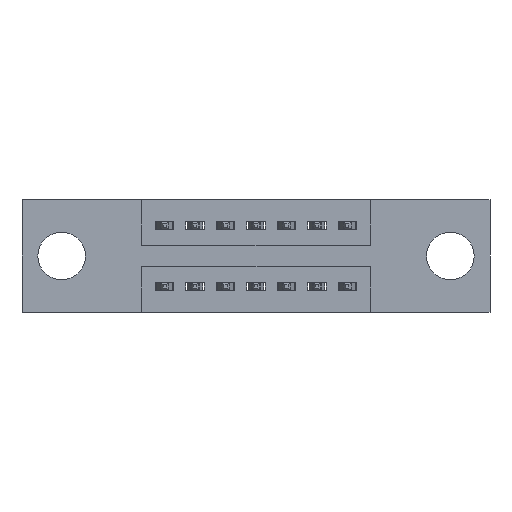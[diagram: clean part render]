
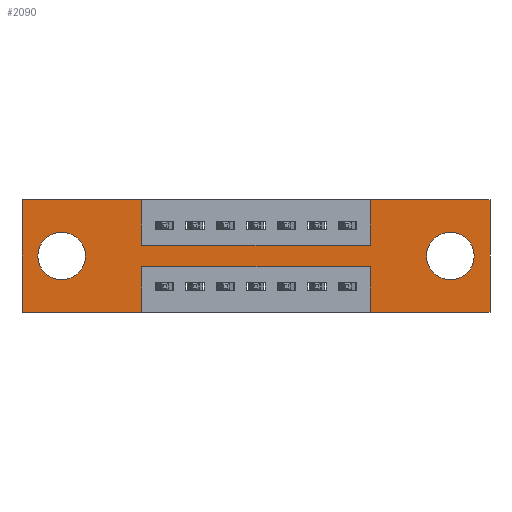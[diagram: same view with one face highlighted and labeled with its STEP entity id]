
A CAD part, front view. The second image highlights one B-rep face of the part: STEP entity #2090.
In plain terms, the highlighted planar face has unit normal (0, -1, 0).
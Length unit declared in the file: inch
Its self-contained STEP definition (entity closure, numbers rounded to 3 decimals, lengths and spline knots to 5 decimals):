
#34 = CARTESIAN_POINT ( 'NONE',  ( 1.535, 0., -0.37 ) ) ;
#132 = EDGE_CURVE ( 'NONE', #414, #5168, #3600, .T. ) ;
#209 = EDGE_CURVE ( 'NONE', #4114, #6818, #6439, .T. ) ;
#267 = DIRECTION ( 'NONE',  ( -1., 0., 0. ) ) ;
#304 = VECTOR ( 'NONE', #3196, 39.37008 ) ;
#315 = DIRECTION ( 'NONE',  ( 0., 0., 1. ) ) ;
#351 = EDGE_CURVE ( 'NONE', #9634, #5052, #2243, .T. ) ;
#364 = AXIS2_PLACEMENT_3D ( 'NONE', #789, #4036, #864 ) ;
#379 = FACE_OUTER_BOUND ( 'NONE', #1907, .T. ) ;
#414 = VERTEX_POINT ( 'NONE', #6142 ) ;
#538 = CARTESIAN_POINT ( 'NONE',  ( 1.1425, 0., 0. ) ) ;
#718 = DIRECTION ( 'NONE',  ( 0., -1., 0. ) ) ;
#789 = CARTESIAN_POINT ( 'NONE',  ( 1.405, 0., -0.185 ) ) ;
#864 = DIRECTION ( 'NONE',  ( 0., 0., -1. ) ) ;
#882 = LINE ( 'NONE', #5283, #1982 ) ;
#901 = DIRECTION ( 'NONE',  ( 0., 1., 0. ) ) ;
#1077 = DIRECTION ( 'NONE',  ( 0., 1., 0. ) ) ;
#1159 = CARTESIAN_POINT ( 'NONE',  ( 0., 0., 0. ) ) ;
#1288 = VECTOR ( 'NONE', #267, 39.37008 ) ;
#1500 = FACE_BOUND ( 'NONE', #8549, .T. ) ;
#1506 = ORIENTED_EDGE ( 'NONE', *, *, #9009, .F. ) ;
#1632 = DIRECTION ( 'NONE',  ( 0., 0., -1. ) ) ;
#1660 = DIRECTION ( 'NONE',  ( 1., 0., 0. ) ) ;
#1853 = CARTESIAN_POINT ( 'NONE',  ( 0.13, 0., -0.185 ) ) ;
#1865 = VECTOR ( 'NONE', #4232, 39.37008 ) ;
#1907 = EDGE_LOOP ( 'NONE', ( #6848, #4354, #9136, #1506, #6352, #5959, #7823, #7233, #10122, #5126, #6548, #6002 ) ) ;
#1982 = VECTOR ( 'NONE', #8779, 39.37008 ) ;
#2044 = LINE ( 'NONE', #6626, #3016 ) ;
#2090 = ADVANCED_FACE ( 'NONE', ( #1500, #10137, #379 ), #10070, .T. ) ;
#2243 = LINE ( 'NONE', #4382, #8785 ) ;
#2335 = CARTESIAN_POINT ( 'NONE',  ( 0.3925, 0., 0. ) ) ;
#2374 = CARTESIAN_POINT ( 'NONE',  ( 1.1425, 0., -0.37 ) ) ;
#2395 = CARTESIAN_POINT ( 'NONE',  ( 1.1425, 0., -0.22 ) ) ;
#2515 = ORIENTED_EDGE ( 'NONE', *, *, #132, .T. ) ;
#2697 = DIRECTION ( 'NONE',  ( 0., 0., 1. ) ) ;
#2710 = CARTESIAN_POINT ( 'NONE',  ( 0.3925, 0., -0.15 ) ) ;
#2835 = CARTESIAN_POINT ( 'NONE',  ( 1.405, 0., -0.263 ) ) ;
#2927 = CIRCLE ( 'NONE', #6636, 0.078 ) ;
#3016 = VECTOR ( 'NONE', #5797, 39.37008 ) ;
#3147 = DIRECTION ( 'NONE',  ( 0., 0., -1. ) ) ;
#3196 = DIRECTION ( 'NONE',  ( 0., 0., 1. ) ) ;
#3208 = LINE ( 'NONE', #3765, #9414 ) ;
#3282 = CIRCLE ( 'NONE', #4840, 0.078 ) ;
#3320 = EDGE_CURVE ( 'NONE', #4879, #5774, #9373, .T. ) ;
#3321 = ORIENTED_EDGE ( 'NONE', *, *, #3840, .T. ) ;
#3591 = LINE ( 'NONE', #8186, #1865 ) ;
#3600 = CIRCLE ( 'NONE', #364, 0.078 ) ;
#3765 = CARTESIAN_POINT ( 'NONE',  ( 0.3925, 0., -0.37 ) ) ;
#3837 = CARTESIAN_POINT ( 'NONE',  ( 0., 0., -0.37 ) ) ;
#3840 = EDGE_CURVE ( 'NONE', #7845, #9971, #7763, .T. ) ;
#3942 = VECTOR ( 'NONE', #9402, 39.37008 ) ;
#3985 = EDGE_CURVE ( 'NONE', #5052, #7646, #9267, .T. ) ;
#4036 = DIRECTION ( 'NONE',  ( 0., 1., 0. ) ) ;
#4043 = ORIENTED_EDGE ( 'NONE', *, *, #4111, .T. ) ;
#4089 = ORIENTED_EDGE ( 'NONE', *, *, #4221, .T. ) ;
#4111 = EDGE_CURVE ( 'NONE', #5168, #414, #3282, .T. ) ;
#4114 = VERTEX_POINT ( 'NONE', #2395 ) ;
#4116 = CARTESIAN_POINT ( 'NONE',  ( 0.3925, 0., -0.22 ) ) ;
#4207 = EDGE_CURVE ( 'NONE', #5157, #8251, #6505, .T. ) ;
#4221 = EDGE_CURVE ( 'NONE', #9971, #7845, #2927, .T. ) ;
#4232 = DIRECTION ( 'NONE',  ( -1., 0., 0. ) ) ;
#4273 = VECTOR ( 'NONE', #1660, 39.37008 ) ;
#4354 = ORIENTED_EDGE ( 'NONE', *, *, #209, .F. ) ;
#4382 = CARTESIAN_POINT ( 'NONE',  ( 0., 0., -0.37 ) ) ;
#4459 = EDGE_CURVE ( 'NONE', #8251, #7363, #5123, .T. ) ;
#4523 = VECTOR ( 'NONE', #2697, 39.37008 ) ;
#4783 = DIRECTION ( 'NONE',  ( 0., 1., 0. ) ) ;
#4819 = CARTESIAN_POINT ( 'NONE',  ( 0.3925, 0., -0.15 ) ) ;
#4840 = AXIS2_PLACEMENT_3D ( 'NONE', #5574, #901, #6359 ) ;
#4864 = CARTESIAN_POINT ( 'NONE',  ( 0.13, 0., -0.107 ) ) ;
#4879 = VERTEX_POINT ( 'NONE', #5333 ) ;
#4888 = VERTEX_POINT ( 'NONE', #538 ) ;
#5052 = VERTEX_POINT ( 'NONE', #5857 ) ;
#5090 = EDGE_CURVE ( 'NONE', #7363, #4888, #2044, .T. ) ;
#5123 = LINE ( 'NONE', #4819, #4273 ) ;
#5126 = ORIENTED_EDGE ( 'NONE', *, *, #8133, .F. ) ;
#5139 = CARTESIAN_POINT ( 'NONE',  ( 0.3925, 0., -0.22 ) ) ;
#5157 = VERTEX_POINT ( 'NONE', #9013 ) ;
#5168 = VERTEX_POINT ( 'NONE', #2835 ) ;
#5258 = DIRECTION ( 'NONE',  ( 0., 0., -1. ) ) ;
#5283 = CARTESIAN_POINT ( 'NONE',  ( 0., 0., 0. ) ) ;
#5333 = CARTESIAN_POINT ( 'NONE',  ( 1.535, 0., 0. ) ) ;
#5454 = CARTESIAN_POINT ( 'NONE',  ( 0., 0., 0. ) ) ;
#5479 = DIRECTION ( 'NONE',  ( 0., 0., -1. ) ) ;
#5574 = CARTESIAN_POINT ( 'NONE',  ( 1.405, 0., -0.185 ) ) ;
#5693 = DIRECTION ( 'NONE',  ( 0., 0., 1. ) ) ;
#5774 = VERTEX_POINT ( 'NONE', #34 ) ;
#5797 = DIRECTION ( 'NONE',  ( 0., 0., 1. ) ) ;
#5812 = EDGE_CURVE ( 'NONE', #7054, #4114, #6093, .T. ) ;
#5857 = CARTESIAN_POINT ( 'NONE',  ( 0., 0., -0.37 ) ) ;
#5890 = CARTESIAN_POINT ( 'NONE',  ( 0.3925, 0., -0.37 ) ) ;
#5959 = ORIENTED_EDGE ( 'NONE', *, *, #9183, .F. ) ;
#6002 = ORIENTED_EDGE ( 'NONE', *, *, #351, .F. ) ;
#6093 = LINE ( 'NONE', #2374, #304 ) ;
#6142 = CARTESIAN_POINT ( 'NONE',  ( 1.405, 0., -0.107 ) ) ;
#6178 = AXIS2_PLACEMENT_3D ( 'NONE', #8085, #4783, #315 ) ;
#6302 = LINE ( 'NONE', #7826, #3942 ) ;
#6352 = ORIENTED_EDGE ( 'NONE', *, *, #3320, .F. ) ;
#6359 = DIRECTION ( 'NONE',  ( 0., 0., -1. ) ) ;
#6439 = LINE ( 'NONE', #4116, #1288 ) ;
#6505 = LINE ( 'NONE', #2335, #9138 ) ;
#6548 = ORIENTED_EDGE ( 'NONE', *, *, #3985, .F. ) ;
#6626 = CARTESIAN_POINT ( 'NONE',  ( 1.1425, 0., 0. ) ) ;
#6636 = AXIS2_PLACEMENT_3D ( 'NONE', #1853, #1077, #5693 ) ;
#6818 = VERTEX_POINT ( 'NONE', #5139 ) ;
#6848 = ORIENTED_EDGE ( 'NONE', *, *, #9260, .F. ) ;
#7054 = VERTEX_POINT ( 'NONE', #9394 ) ;
#7233 = ORIENTED_EDGE ( 'NONE', *, *, #4459, .F. ) ;
#7363 = VERTEX_POINT ( 'NONE', #8159 ) ;
#7420 = DIRECTION ( 'NONE',  ( -1., 0., 0. ) ) ;
#7646 = VERTEX_POINT ( 'NONE', #5454 ) ;
#7743 = VECTOR ( 'NONE', #5258, 39.37008 ) ;
#7763 = CIRCLE ( 'NONE', #6178, 0.078 ) ;
#7823 = ORIENTED_EDGE ( 'NONE', *, *, #5090, .F. ) ;
#7826 = CARTESIAN_POINT ( 'NONE',  ( 0., 0., 0. ) ) ;
#7845 = VERTEX_POINT ( 'NONE', #4864 ) ;
#7900 = AXIS2_PLACEMENT_3D ( 'NONE', #3837, #718, #3147 ) ;
#8085 = CARTESIAN_POINT ( 'NONE',  ( 0.13, 0., -0.185 ) ) ;
#8133 = EDGE_CURVE ( 'NONE', #7646, #5157, #882, .T. ) ;
#8159 = CARTESIAN_POINT ( 'NONE',  ( 1.1425, 0., -0.15 ) ) ;
#8186 = CARTESIAN_POINT ( 'NONE',  ( 0., 0., -0.37 ) ) ;
#8251 = VERTEX_POINT ( 'NONE', #2710 ) ;
#8470 = CARTESIAN_POINT ( 'NONE',  ( 0.13, 0., -0.263 ) ) ;
#8496 = EDGE_LOOP ( 'NONE', ( #3321, #4089 ) ) ;
#8549 = EDGE_LOOP ( 'NONE', ( #2515, #4043 ) ) ;
#8779 = DIRECTION ( 'NONE',  ( 1., 0., 0. ) ) ;
#8785 = VECTOR ( 'NONE', #7420, 39.37008 ) ;
#9009 = EDGE_CURVE ( 'NONE', #5774, #7054, #3591, .T. ) ;
#9013 = CARTESIAN_POINT ( 'NONE',  ( 0.3925, 0., 0. ) ) ;
#9136 = ORIENTED_EDGE ( 'NONE', *, *, #5812, .F. ) ;
#9138 = VECTOR ( 'NONE', #1632, 39.37008 ) ;
#9183 = EDGE_CURVE ( 'NONE', #4888, #4879, #6302, .T. ) ;
#9220 = CARTESIAN_POINT ( 'NONE',  ( 1.535, 0., 0. ) ) ;
#9260 = EDGE_CURVE ( 'NONE', #6818, #9634, #3208, .T. ) ;
#9267 = LINE ( 'NONE', #1159, #4523 ) ;
#9373 = LINE ( 'NONE', #9220, #7743 ) ;
#9394 = CARTESIAN_POINT ( 'NONE',  ( 1.1425, 0., -0.37 ) ) ;
#9402 = DIRECTION ( 'NONE',  ( 1., 0., 0. ) ) ;
#9414 = VECTOR ( 'NONE', #5479, 39.37008 ) ;
#9634 = VERTEX_POINT ( 'NONE', #5890 ) ;
#9971 = VERTEX_POINT ( 'NONE', #8470 ) ;
#10070 = PLANE ( 'NONE',  #7900 ) ;
#10122 = ORIENTED_EDGE ( 'NONE', *, *, #4207, .F. ) ;
#10137 = FACE_BOUND ( 'NONE', #8496, .T. ) ;
